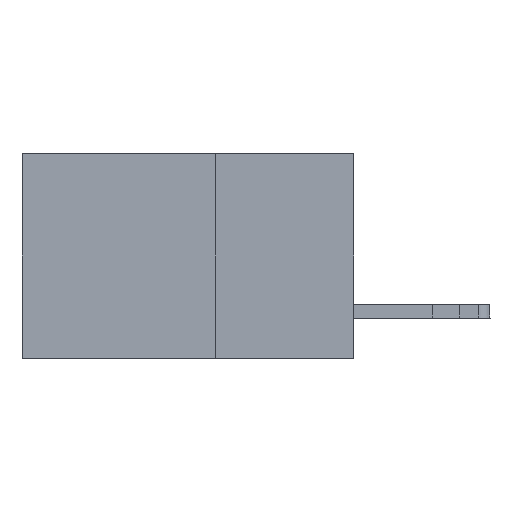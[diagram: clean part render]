
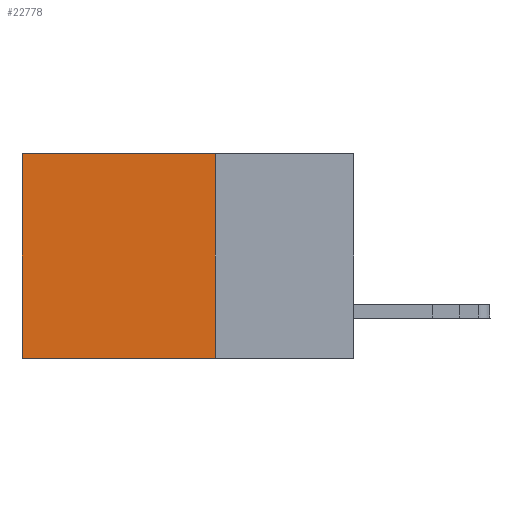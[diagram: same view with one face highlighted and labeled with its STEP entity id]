
A CAD part, left-side view. The second image highlights one B-rep face of the part: STEP entity #22778.
In plain terms, the highlighted planar face has unit normal (-1, 0, 0).
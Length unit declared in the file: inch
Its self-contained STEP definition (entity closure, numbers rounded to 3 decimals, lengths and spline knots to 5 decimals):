
#464 = ORIENTED_EDGE ( 'NONE', *, *, #33786, .T. ) ;
#1499 = CARTESIAN_POINT ( 'NONE',  ( 0.2875, 0.25, 0. ) ) ;
#1892 = DIRECTION ( 'NONE',  ( 0., 1., 0. ) ) ;
#2972 = LINE ( 'NONE', #23738, #31518 ) ;
#3621 = VERTEX_POINT ( 'NONE', #16822 ) ;
#3858 = PLANE ( 'NONE',  #19110 ) ;
#4128 = CARTESIAN_POINT ( 'NONE',  ( 0.2875, 0.25, 0. ) ) ;
#5747 = ORIENTED_EDGE ( 'NONE', *, *, #10030, .F. ) ;
#7468 = VECTOR ( 'NONE', #1892, 39.37008 ) ;
#9426 = DIRECTION ( 'NONE',  ( 0., 0., -1. ) ) ;
#10030 = EDGE_CURVE ( 'NONE', #30534, #25800, #19205, .T. ) ;
#10671 = CARTESIAN_POINT ( 'NONE',  ( 0.2875, 0.25, 0. ) ) ;
#11994 = CARTESIAN_POINT ( 'NONE',  ( 0.2875, 0.25, -0.37 ) ) ;
#14565 = ORIENTED_EDGE ( 'NONE', *, *, #32710, .T. ) ;
#14934 = EDGE_LOOP ( 'NONE', ( #464, #19587, #5747, #14565 ) ) ;
#15814 = DIRECTION ( 'NONE',  ( 1., 0., 0. ) ) ;
#16239 = CARTESIAN_POINT ( 'NONE',  ( 0.2875, 0.25, 0. ) ) ;
#16392 = DIRECTION ( 'NONE',  ( 0., 0., -1. ) ) ;
#16822 = CARTESIAN_POINT ( 'NONE',  ( 0.2875, 0.6, -0.37 ) ) ;
#18960 = CARTESIAN_POINT ( 'NONE',  ( 0.2875, 0.6, 0. ) ) ;
#19110 = AXIS2_PLACEMENT_3D ( 'NONE', #1499, #15814, #16392 ) ;
#19205 = LINE ( 'NONE', #4128, #33829 ) ;
#19301 = VERTEX_POINT ( 'NONE', #18960 ) ;
#19587 = ORIENTED_EDGE ( 'NONE', *, *, #21598, .F. ) ;
#21598 = EDGE_CURVE ( 'NONE', #25800, #3621, #34427, .T. ) ;
#22778 = ADVANCED_FACE ( 'NONE', ( #31287 ), #3858, .F. ) ;
#23738 = CARTESIAN_POINT ( 'NONE',  ( 0.2875, 0.6, 0. ) ) ;
#25430 = LINE ( 'NONE', #16239, #29551 ) ;
#25800 = VERTEX_POINT ( 'NONE', #36687 ) ;
#29551 = VECTOR ( 'NONE', #30918, 39.37008 ) ;
#30534 = VERTEX_POINT ( 'NONE', #10671 ) ;
#30918 = DIRECTION ( 'NONE',  ( 0., 1., 0. ) ) ;
#31171 = DIRECTION ( 'NONE',  ( 0., 0., -1. ) ) ;
#31287 = FACE_OUTER_BOUND ( 'NONE', #14934, .T. ) ;
#31518 = VECTOR ( 'NONE', #9426, 39.37008 ) ;
#32710 = EDGE_CURVE ( 'NONE', #30534, #19301, #25430, .T. ) ;
#33786 = EDGE_CURVE ( 'NONE', #19301, #3621, #2972, .T. ) ;
#33829 = VECTOR ( 'NONE', #31171, 39.37008 ) ;
#34427 = LINE ( 'NONE', #11994, #7468 ) ;
#36687 = CARTESIAN_POINT ( 'NONE',  ( 0.2875, 0.25, -0.37 ) ) ;
